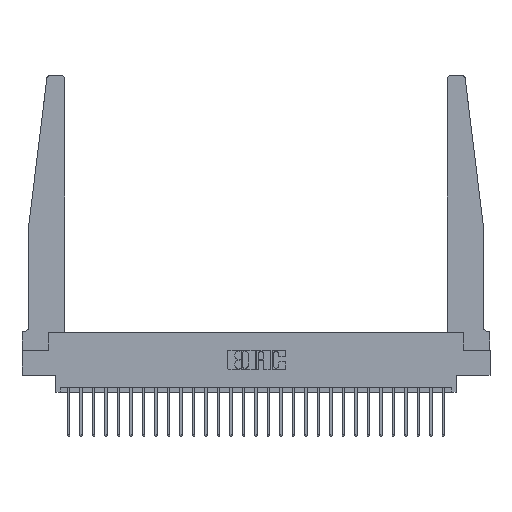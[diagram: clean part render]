
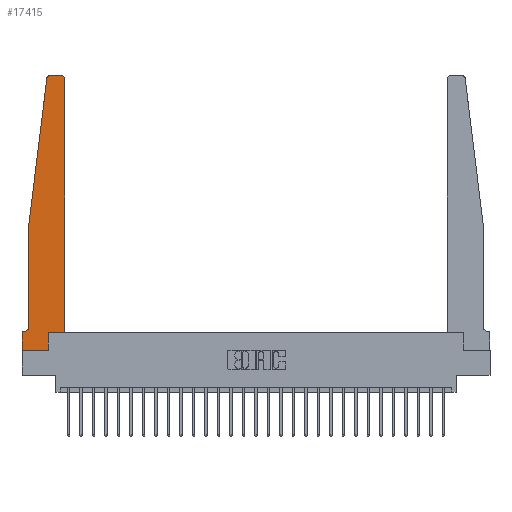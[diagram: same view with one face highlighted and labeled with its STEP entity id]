
A CAD part, top view. The second image highlights one B-rep face of the part: STEP entity #17415.
In plain terms, the highlighted planar face has unit normal (0, 0, 1).
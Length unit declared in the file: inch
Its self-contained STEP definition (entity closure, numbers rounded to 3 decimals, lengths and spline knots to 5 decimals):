
#404 = CARTESIAN_POINT ( 'NONE',  ( 0.395, 2.75, 0.37 ) ) ;
#677 = EDGE_CURVE ( 'NONE', #19684, #20192, #12416, .T. ) ;
#1572 = CARTESIAN_POINT ( 'NONE',  ( 0., 0., 0.37 ) ) ;
#1638 = CARTESIAN_POINT ( 'NONE',  ( 0.065, 0.2375, 0.37 ) ) ;
#1763 = DIRECTION ( 'NONE',  ( 0., -1., 0. ) ) ;
#1897 = CARTESIAN_POINT ( 'NONE',  ( 0., 0., 0.37 ) ) ;
#1951 = LINE ( 'NONE', #8230, #9149 ) ;
#2000 = VERTEX_POINT ( 'NONE', #6932 ) ;
#2337 = EDGE_LOOP ( 'NONE', ( #10464, #22431, #5598, #4644, #12724, #27011, #4973, #19946, #9667, #5769, #25669, #22556 ) ) ;
#2573 = CIRCLE ( 'NONE', #13913, 0.03 ) ;
#2859 = VERTEX_POINT ( 'NONE', #13418 ) ;
#3623 = CARTESIAN_POINT ( 'NONE',  ( 0., 0.1875, 0.37 ) ) ;
#3911 = VECTOR ( 'NONE', #12252, 39.37008 ) ;
#4401 = DIRECTION ( 'NONE',  ( 0., 0., 1. ) ) ;
#4644 = ORIENTED_EDGE ( 'NONE', *, *, #10265, .T. ) ;
#4670 = DIRECTION ( 'NONE',  ( 0., -1., 0. ) ) ;
#4759 = VERTEX_POINT ( 'NONE', #20420 ) ;
#4973 = ORIENTED_EDGE ( 'NONE', *, *, #12057, .T. ) ;
#5598 = ORIENTED_EDGE ( 'NONE', *, *, #677, .T. ) ;
#5624 = EDGE_CURVE ( 'NONE', #4759, #26376, #10065, .T. ) ;
#5769 = ORIENTED_EDGE ( 'NONE', *, *, #15264, .T. ) ;
#6314 = CARTESIAN_POINT ( 'NONE',  ( 0., 0.1875, 0.37 ) ) ;
#6932 = CARTESIAN_POINT ( 'NONE',  ( 0.2605, 0., 0.37 ) ) ;
#7069 = EDGE_CURVE ( 'NONE', #16665, #19684, #2573, .T. ) ;
#7172 = CARTESIAN_POINT ( 'NONE',  ( 0.065, 1.25, 0.37 ) ) ;
#8043 = DIRECTION ( 'NONE',  ( 0., 0., 1. ) ) ;
#8230 = CARTESIAN_POINT ( 'NONE',  ( 0., 0., 0.37 ) ) ;
#8448 = CARTESIAN_POINT ( 'NONE',  ( 0.2605, 0.18, 0.37 ) ) ;
#8562 = CARTESIAN_POINT ( 'NONE',  ( 0.27653, 2.72, 0.37 ) ) ;
#8581 = LINE ( 'NONE', #22989, #10904 ) ;
#8720 = EDGE_CURVE ( 'NONE', #16803, #2000, #1951, .T. ) ;
#9149 = VECTOR ( 'NONE', #24690, 39.37008 ) ;
#9667 = ORIENTED_EDGE ( 'NONE', *, *, #12062, .T. ) ;
#9799 = CARTESIAN_POINT ( 'NONE',  ( 0.065, 0.1875, 0.37 ) ) ;
#10065 = LINE ( 'NONE', #9799, #13013 ) ;
#10265 = EDGE_CURVE ( 'NONE', #20192, #18980, #21258, .T. ) ;
#10464 = ORIENTED_EDGE ( 'NONE', *, *, #14505, .T. ) ;
#10558 = PLANE ( 'NONE',  #10575 ) ;
#10575 = AXIS2_PLACEMENT_3D ( 'NONE', #6314, #4401, #15184 ) ;
#10673 = VERTEX_POINT ( 'NONE', #404 ) ;
#10904 = VECTOR ( 'NONE', #14607, 39.37008 ) ;
#10975 = EDGE_CURVE ( 'NONE', #19526, #14811, #16781, .T. ) ;
#11321 = VECTOR ( 'NONE', #4670, 39.37008 ) ;
#12057 = EDGE_CURVE ( 'NONE', #26376, #16803, #14470, .T. ) ;
#12062 = EDGE_CURVE ( 'NONE', #2000, #2859, #16538, .T. ) ;
#12252 = DIRECTION ( 'NONE',  ( 0., 1., 0. ) ) ;
#12416 = LINE ( 'NONE', #18590, #18123 ) ;
#12724 = ORIENTED_EDGE ( 'NONE', *, *, #25660, .T. ) ;
#12932 = DIRECTION ( 'NONE',  ( 0., 0., 1. ) ) ;
#13013 = VECTOR ( 'NONE', #26805, 39.37008 ) ;
#13418 = CARTESIAN_POINT ( 'NONE',  ( 0.2605, 0.18, 0.37 ) ) ;
#13867 = AXIS2_PLACEMENT_3D ( 'NONE', #19143, #22867, #14621 ) ;
#13913 = AXIS2_PLACEMENT_3D ( 'NONE', #8562, #12932, #19110 ) ;
#14127 = LINE ( 'NONE', #18130, #21871 ) ;
#14470 = LINE ( 'NONE', #1897, #21464 ) ;
#14473 = EDGE_CURVE ( 'NONE', #14811, #10673, #19217, .T. ) ;
#14505 = EDGE_CURVE ( 'NONE', #10673, #16665, #8581, .T. ) ;
#14607 = DIRECTION ( 'NONE',  ( -1., 0., 0. ) ) ;
#14621 = DIRECTION ( 'NONE',  ( -1., 0., 0. ) ) ;
#14811 = VERTEX_POINT ( 'NONE', #20483 ) ;
#15184 = DIRECTION ( 'NONE',  ( 1., 0., 0. ) ) ;
#15264 = EDGE_CURVE ( 'NONE', #2859, #19526, #14127, .T. ) ;
#16396 = DIRECTION ( 'NONE',  ( 1., 0., 0. ) ) ;
#16538 = LINE ( 'NONE', #8448, #26706 ) ;
#16665 = VERTEX_POINT ( 'NONE', #18007 ) ;
#16781 = LINE ( 'NONE', #20889, #3911 ) ;
#16803 = VERTEX_POINT ( 'NONE', #1572 ) ;
#16945 = CARTESIAN_POINT ( 'NONE',  ( 0.24675, 2.72367, 0.37 ) ) ;
#16996 = FACE_OUTER_BOUND ( 'NONE', #2337, .T. ) ;
#17415 = ADVANCED_FACE ( 'NONE', ( #16996 ), #10558, .T. ) ;
#18007 = CARTESIAN_POINT ( 'NONE',  ( 0.27653, 2.75, 0.37 ) ) ;
#18123 = VECTOR ( 'NONE', #26960, 39.37008 ) ;
#18130 = CARTESIAN_POINT ( 'NONE',  ( 0.425, 0.18, 0.37 ) ) ;
#18590 = CARTESIAN_POINT ( 'NONE',  ( 0.065, 1.25, 0.37 ) ) ;
#18799 = AXIS2_PLACEMENT_3D ( 'NONE', #26830, #8043, #16396 ) ;
#18980 = VERTEX_POINT ( 'NONE', #1638 ) ;
#19110 = DIRECTION ( 'NONE',  ( 1., 0., 0. ) ) ;
#19143 = CARTESIAN_POINT ( 'NONE',  ( 0.015, 0.2375, 0.37 ) ) ;
#19217 = CIRCLE ( 'NONE', #18799, 0.03 ) ;
#19526 = VERTEX_POINT ( 'NONE', #21203 ) ;
#19684 = VERTEX_POINT ( 'NONE', #16945 ) ;
#19946 = ORIENTED_EDGE ( 'NONE', *, *, #8720, .T. ) ;
#20192 = VERTEX_POINT ( 'NONE', #7172 ) ;
#20420 = CARTESIAN_POINT ( 'NONE',  ( 0.015, 0.1875, 0.37 ) ) ;
#20483 = CARTESIAN_POINT ( 'NONE',  ( 0.425, 2.72, 0.37 ) ) ;
#20889 = CARTESIAN_POINT ( 'NONE',  ( 0.425, 0.18, 0.37 ) ) ;
#20992 = CARTESIAN_POINT ( 'NONE',  ( 0.065, 1.25, 0.37 ) ) ;
#21203 = CARTESIAN_POINT ( 'NONE',  ( 0.425, 0.18, 0.37 ) ) ;
#21258 = LINE ( 'NONE', #20992, #11321 ) ;
#21464 = VECTOR ( 'NONE', #1763, 39.37008 ) ;
#21871 = VECTOR ( 'NONE', #22378, 39.37008 ) ;
#22378 = DIRECTION ( 'NONE',  ( 1., 0., 0. ) ) ;
#22431 = ORIENTED_EDGE ( 'NONE', *, *, #7069, .T. ) ;
#22556 = ORIENTED_EDGE ( 'NONE', *, *, #14473, .T. ) ;
#22867 = DIRECTION ( 'NONE',  ( 0., 0., -1. ) ) ;
#22989 = CARTESIAN_POINT ( 'NONE',  ( 0.25, 2.75, 0.37 ) ) ;
#24690 = DIRECTION ( 'NONE',  ( 1., 0., 0. ) ) ;
#24912 = DIRECTION ( 'NONE',  ( 0., 1., 0. ) ) ;
#25660 = EDGE_CURVE ( 'NONE', #18980, #4759, #27036, .T. ) ;
#25669 = ORIENTED_EDGE ( 'NONE', *, *, #10975, .T. ) ;
#26376 = VERTEX_POINT ( 'NONE', #3623 ) ;
#26706 = VECTOR ( 'NONE', #24912, 39.37008 ) ;
#26805 = DIRECTION ( 'NONE',  ( -1., 0., 0. ) ) ;
#26830 = CARTESIAN_POINT ( 'NONE',  ( 0.395, 2.72, 0.37 ) ) ;
#26960 = DIRECTION ( 'NONE',  ( -0.122, -0.992, 0. ) ) ;
#27011 = ORIENTED_EDGE ( 'NONE', *, *, #5624, .T. ) ;
#27036 = CIRCLE ( 'NONE', #13867, 0.05 ) ;
